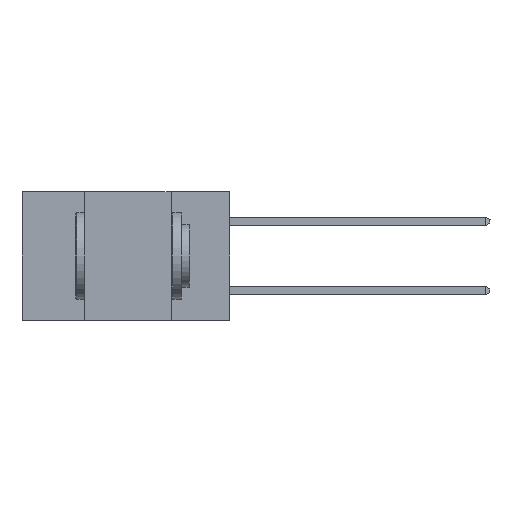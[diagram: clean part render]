
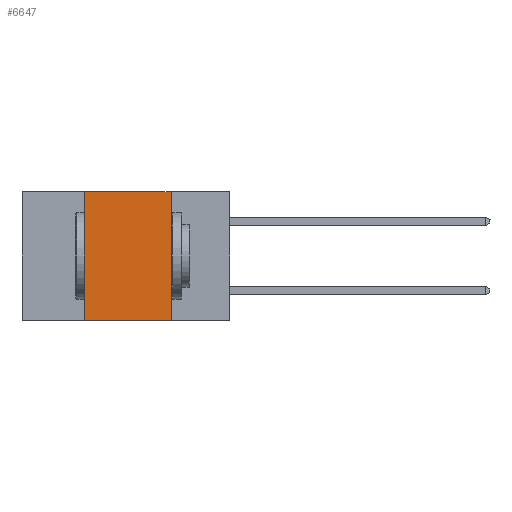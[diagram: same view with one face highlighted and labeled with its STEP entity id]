
A CAD part, left-side view. The second image highlights one B-rep face of the part: STEP entity #6647.
In plain terms, the highlighted planar face has unit normal (-1, 0, 0).
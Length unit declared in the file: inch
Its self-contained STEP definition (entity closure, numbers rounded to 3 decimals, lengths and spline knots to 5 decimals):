
#97 = EDGE_CURVE ( 'NONE', #1431, #735, #8505, .T. ) ;
#130 = DIRECTION ( 'NONE',  ( 0., 0., 1. ) ) ;
#253 = ORIENTED_EDGE ( 'NONE', *, *, #4902, .F. ) ;
#658 = CARTESIAN_POINT ( 'NONE',  ( 0., 0.17, -0.37 ) ) ;
#735 = VERTEX_POINT ( 'NONE', #3949 ) ;
#835 = CARTESIAN_POINT ( 'NONE',  ( 0., 0.42, 0. ) ) ;
#839 = LINE ( 'NONE', #6604, #3770 ) ;
#1126 = VERTEX_POINT ( 'NONE', #835 ) ;
#1431 = VERTEX_POINT ( 'NONE', #4737 ) ;
#1441 = PLANE ( 'NONE',  #7112 ) ;
#1516 = LINE ( 'NONE', #2801, #2737 ) ;
#1641 = ORIENTED_EDGE ( 'NONE', *, *, #8178, .F. ) ;
#1698 = VECTOR ( 'NONE', #9015, 39.37008 ) ;
#1995 = CARTESIAN_POINT ( 'NONE',  ( 0., 0.6, -0.37 ) ) ;
#2201 = LINE ( 'NONE', #658, #4903 ) ;
#2735 = DIRECTION ( 'NONE',  ( 0., 0., -1. ) ) ;
#2737 = VECTOR ( 'NONE', #7220, 39.37008 ) ;
#2801 = CARTESIAN_POINT ( 'NONE',  ( 0., 0.6, 0. ) ) ;
#3602 = FACE_OUTER_BOUND ( 'NONE', #4421, .T. ) ;
#3627 = ORIENTED_EDGE ( 'NONE', *, *, #8981, .F. ) ;
#3770 = VECTOR ( 'NONE', #130, 39.37008 ) ;
#3949 = CARTESIAN_POINT ( 'NONE',  ( 0., 0.17, -0.37 ) ) ;
#4421 = EDGE_LOOP ( 'NONE', ( #3627, #1641, #253, #7772 ) ) ;
#4593 = DIRECTION ( 'NONE',  ( 1., 0., 0. ) ) ;
#4613 = CARTESIAN_POINT ( 'NONE',  ( 0., 0.17, 0. ) ) ;
#4737 = CARTESIAN_POINT ( 'NONE',  ( 0., 0.42, -0.37 ) ) ;
#4902 = EDGE_CURVE ( 'NONE', #1431, #1126, #839, .T. ) ;
#4903 = VECTOR ( 'NONE', #2735, 39.37008 ) ;
#6039 = CARTESIAN_POINT ( 'NONE',  ( 0., 0.6, 0. ) ) ;
#6433 = VERTEX_POINT ( 'NONE', #4613 ) ;
#6604 = CARTESIAN_POINT ( 'NONE',  ( 0., 0.42, -0.37 ) ) ;
#6647 = ADVANCED_FACE ( 'NONE', ( #3602 ), #1441, .F. ) ;
#7112 = AXIS2_PLACEMENT_3D ( 'NONE', #6039, #4593, #7186 ) ;
#7186 = DIRECTION ( 'NONE',  ( 0., 0., -1. ) ) ;
#7220 = DIRECTION ( 'NONE',  ( 0., -1., 0. ) ) ;
#7772 = ORIENTED_EDGE ( 'NONE', *, *, #97, .T. ) ;
#8178 = EDGE_CURVE ( 'NONE', #1126, #6433, #1516, .T. ) ;
#8505 = LINE ( 'NONE', #1995, #1698 ) ;
#8981 = EDGE_CURVE ( 'NONE', #6433, #735, #2201, .T. ) ;
#9015 = DIRECTION ( 'NONE',  ( 0., -1., 0. ) ) ;
